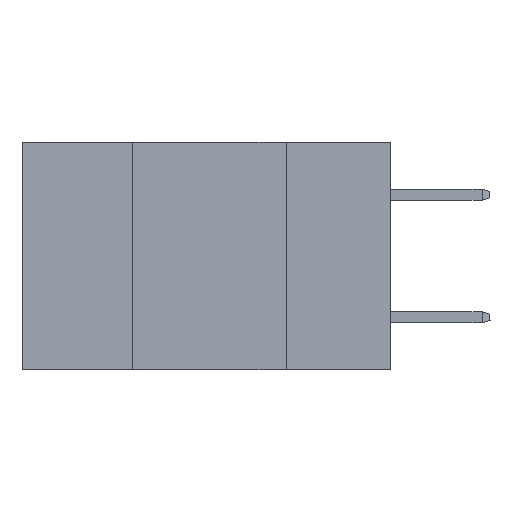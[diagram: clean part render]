
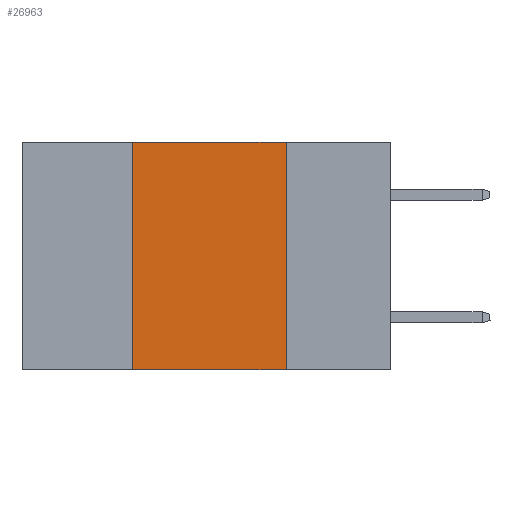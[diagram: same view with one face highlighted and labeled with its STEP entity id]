
A CAD part, left-side view. The second image highlights one B-rep face of the part: STEP entity #26963.
In plain terms, the highlighted planar face has unit normal (-1, 0, 0).
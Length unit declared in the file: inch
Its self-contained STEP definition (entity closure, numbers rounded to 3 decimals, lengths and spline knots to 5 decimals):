
#242 = LINE ( 'NONE', #34710, #4168 ) ;
#1175 = EDGE_LOOP ( 'NONE', ( #27770, #15906, #30849, #37800 ) ) ;
#4168 = VECTOR ( 'NONE', #31804, 39.37008 ) ;
#6452 = DIRECTION ( 'NONE',  ( 0., 0., 1. ) ) ;
#7060 = CARTESIAN_POINT ( 'NONE',  ( 0., 0.42, 0. ) ) ;
#8741 = VERTEX_POINT ( 'NONE', #30227 ) ;
#10878 = EDGE_CURVE ( 'NONE', #25025, #25789, #34931, .T. ) ;
#10973 = CARTESIAN_POINT ( 'NONE',  ( 0., 0.6, 0. ) ) ;
#10984 = EDGE_CURVE ( 'NONE', #25789, #32150, #32424, .T. ) ;
#11617 = DIRECTION ( 'NONE',  ( 0., 0., -1. ) ) ;
#12411 = VECTOR ( 'NONE', #21708, 39.37008 ) ;
#13901 = FACE_OUTER_BOUND ( 'NONE', #1175, .T. ) ;
#14566 = CARTESIAN_POINT ( 'NONE',  ( 0., 0.17, 0. ) ) ;
#14921 = LINE ( 'NONE', #18419, #12411 ) ;
#15906 = ORIENTED_EDGE ( 'NONE', *, *, #10984, .F. ) ;
#16712 = VECTOR ( 'NONE', #6452, 39.37008 ) ;
#18403 = CARTESIAN_POINT ( 'NONE',  ( 0., 0.42, 0. ) ) ;
#18419 = CARTESIAN_POINT ( 'NONE',  ( 0., 0.17, 0. ) ) ;
#19591 = AXIS2_PLACEMENT_3D ( 'NONE', #36779, #34445, #11617 ) ;
#20372 = EDGE_CURVE ( 'NONE', #25025, #8741, #242, .T. ) ;
#21708 = DIRECTION ( 'NONE',  ( 0., 0., -1. ) ) ;
#25025 = VERTEX_POINT ( 'NONE', #26837 ) ;
#25789 = VERTEX_POINT ( 'NONE', #18403 ) ;
#26837 = CARTESIAN_POINT ( 'NONE',  ( 0., 0.42, -0.37 ) ) ;
#26963 = ADVANCED_FACE ( 'NONE', ( #13901 ), #30170, .F. ) ;
#27770 = ORIENTED_EDGE ( 'NONE', *, *, #29708, .F. ) ;
#29708 = EDGE_CURVE ( 'NONE', #32150, #8741, #14921, .T. ) ;
#30170 = PLANE ( 'NONE',  #19591 ) ;
#30227 = CARTESIAN_POINT ( 'NONE',  ( 0., 0.17, -0.37 ) ) ;
#30849 = ORIENTED_EDGE ( 'NONE', *, *, #10878, .F. ) ;
#31804 = DIRECTION ( 'NONE',  ( 0., -1., 0. ) ) ;
#32150 = VERTEX_POINT ( 'NONE', #14566 ) ;
#32424 = LINE ( 'NONE', #10973, #39090 ) ;
#34445 = DIRECTION ( 'NONE',  ( 1., 0., 0. ) ) ;
#34710 = CARTESIAN_POINT ( 'NONE',  ( 0., 0.6, -0.37 ) ) ;
#34931 = LINE ( 'NONE', #7060, #16712 ) ;
#36779 = CARTESIAN_POINT ( 'NONE',  ( 0., 0.6, 0. ) ) ;
#37800 = ORIENTED_EDGE ( 'NONE', *, *, #20372, .T. ) ;
#39090 = VECTOR ( 'NONE', #39430, 39.37008 ) ;
#39430 = DIRECTION ( 'NONE',  ( 0., -1., 0. ) ) ;
